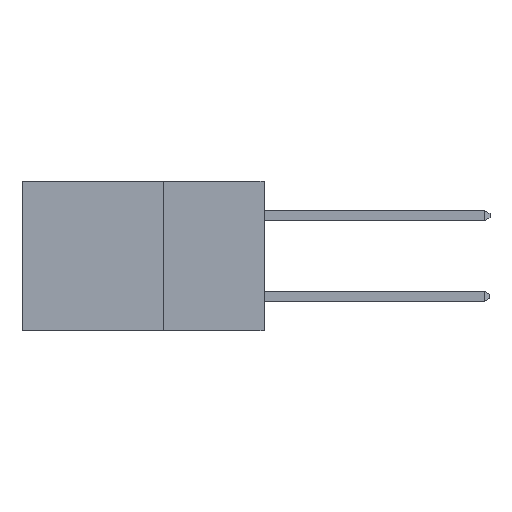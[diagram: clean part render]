
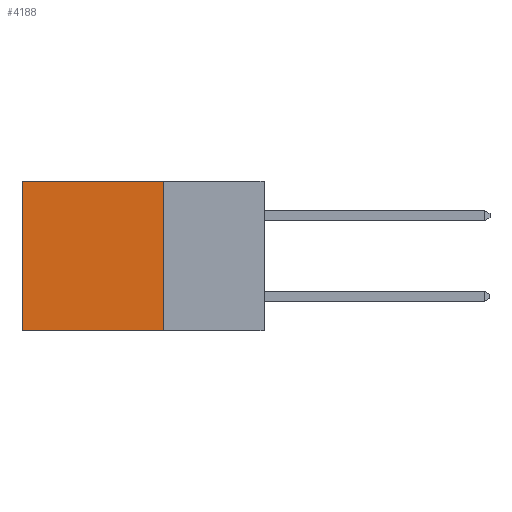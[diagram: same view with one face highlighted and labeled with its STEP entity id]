
A CAD part, left-side view. The second image highlights one B-rep face of the part: STEP entity #4188.
In plain terms, the highlighted planar face has unit normal (-1, 0, 0).
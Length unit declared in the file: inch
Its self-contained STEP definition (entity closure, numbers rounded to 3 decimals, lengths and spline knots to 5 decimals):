
#367 = AXIS2_PLACEMENT_3D ( 'NONE', #485, #4943, #4027 ) ;
#386 = CARTESIAN_POINT ( 'NONE',  ( 0.2615, 0.25, 0. ) ) ;
#485 = CARTESIAN_POINT ( 'NONE',  ( 0.2615, 0.25, -0.37 ) ) ;
#1509 = CARTESIAN_POINT ( 'NONE',  ( 0.2615, 0.25, 0. ) ) ;
#1740 = EDGE_CURVE ( 'NONE', #7438, #2967, #11099, .T. ) ;
#2233 = LINE ( 'NONE', #386, #4095 ) ;
#2510 = CARTESIAN_POINT ( 'NONE',  ( 0.2615, 0.6, -0.37 ) ) ;
#2646 = ORIENTED_EDGE ( 'NONE', *, *, #9415, .T. ) ;
#2967 = VERTEX_POINT ( 'NONE', #4256 ) ;
#3045 = DIRECTION ( 'NONE',  ( 0., 1., 0. ) ) ;
#3682 = FACE_OUTER_BOUND ( 'NONE', #5959, .T. ) ;
#4027 = DIRECTION ( 'NONE',  ( 0., 0., -1. ) ) ;
#4095 = VECTOR ( 'NONE', #3045, 39.37008 ) ;
#4188 = ADVANCED_FACE ( 'NONE', ( #3682 ), #4649, .F. ) ;
#4256 = CARTESIAN_POINT ( 'NONE',  ( 0.2615, 0.25, -0.37 ) ) ;
#4432 = ORIENTED_EDGE ( 'NONE', *, *, #11037, .F. ) ;
#4649 = PLANE ( 'NONE',  #367 ) ;
#4943 = DIRECTION ( 'NONE',  ( 1., 0., 0. ) ) ;
#5353 = LINE ( 'NONE', #8937, #8598 ) ;
#5749 = LINE ( 'NONE', #8247, #10441 ) ;
#5959 = EDGE_LOOP ( 'NONE', ( #2646, #4432, #7772, #7565 ) ) ;
#7438 = VERTEX_POINT ( 'NONE', #1509 ) ;
#7565 = ORIENTED_EDGE ( 'NONE', *, *, #8230, .T. ) ;
#7772 = ORIENTED_EDGE ( 'NONE', *, *, #1740, .F. ) ;
#8061 = VERTEX_POINT ( 'NONE', #2510 ) ;
#8230 = EDGE_CURVE ( 'NONE', #7438, #10493, #2233, .T. ) ;
#8247 = CARTESIAN_POINT ( 'NONE',  ( 0.2615, 0.6, -0.37 ) ) ;
#8562 = VECTOR ( 'NONE', #10259, 39.37008 ) ;
#8598 = VECTOR ( 'NONE', #8880, 39.37008 ) ;
#8880 = DIRECTION ( 'NONE',  ( 0., 1., 0. ) ) ;
#8937 = CARTESIAN_POINT ( 'NONE',  ( 0.2615, 0.25, -0.37 ) ) ;
#9205 = DIRECTION ( 'NONE',  ( 0., 0., -1. ) ) ;
#9415 = EDGE_CURVE ( 'NONE', #10493, #8061, #5749, .T. ) ;
#10066 = CARTESIAN_POINT ( 'NONE',  ( 0.2615, 0.6, 0. ) ) ;
#10259 = DIRECTION ( 'NONE',  ( 0., 0., -1. ) ) ;
#10313 = CARTESIAN_POINT ( 'NONE',  ( 0.2615, 0.25, -0.37 ) ) ;
#10441 = VECTOR ( 'NONE', #9205, 39.37008 ) ;
#10493 = VERTEX_POINT ( 'NONE', #10066 ) ;
#11037 = EDGE_CURVE ( 'NONE', #2967, #8061, #5353, .T. ) ;
#11099 = LINE ( 'NONE', #10313, #8562 ) ;
